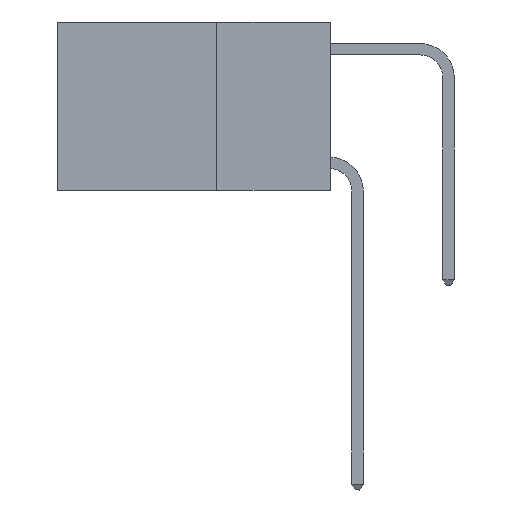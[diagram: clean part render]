
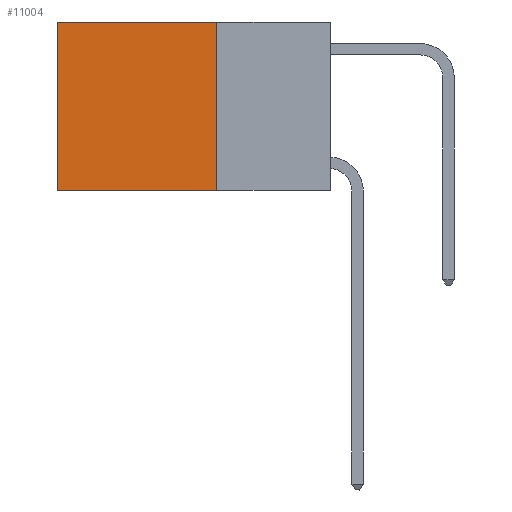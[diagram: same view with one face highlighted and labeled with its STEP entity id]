
A CAD part, left-side view. The second image highlights one B-rep face of the part: STEP entity #11004.
In plain terms, the highlighted planar face has unit normal (-1, 0, 0).
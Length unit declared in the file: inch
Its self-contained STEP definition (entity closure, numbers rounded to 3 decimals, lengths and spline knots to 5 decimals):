
#672 = DIRECTION ( 'NONE',  ( 0., 1., 0. ) ) ;
#1642 = DIRECTION ( 'NONE',  ( 0., 0., -1. ) ) ;
#2184 = VECTOR ( 'NONE', #5513, 39.37008 ) ;
#2373 = VECTOR ( 'NONE', #6377, 39.37008 ) ;
#2570 = PLANE ( 'NONE',  #9098 ) ;
#2979 = VECTOR ( 'NONE', #1642, 39.37008 ) ;
#3345 = VERTEX_POINT ( 'NONE', #8348 ) ;
#3368 = CARTESIAN_POINT ( 'NONE',  ( 0.2625, 0.6, 0. ) ) ;
#3520 = VERTEX_POINT ( 'NONE', #6360 ) ;
#3908 = ORIENTED_EDGE ( 'NONE', *, *, #7059, .F. ) ;
#4162 = EDGE_LOOP ( 'NONE', ( #11677, #3908, #10853, #10367 ) ) ;
#4554 = CARTESIAN_POINT ( 'NONE',  ( 0.2625, 0.6, 0. ) ) ;
#5513 = DIRECTION ( 'NONE',  ( 0., 0., -1. ) ) ;
#5763 = CARTESIAN_POINT ( 'NONE',  ( 0.2625, 0.25, 0. ) ) ;
#5801 = LINE ( 'NONE', #6273, #2979 ) ;
#6016 = EDGE_CURVE ( 'NONE', #13277, #3520, #5801, .T. ) ;
#6273 = CARTESIAN_POINT ( 'NONE',  ( 0.2625, 0.25, 0. ) ) ;
#6360 = CARTESIAN_POINT ( 'NONE',  ( 0.2625, 0.25, -0.37 ) ) ;
#6377 = DIRECTION ( 'NONE',  ( 0., 1., 0. ) ) ;
#6893 = CARTESIAN_POINT ( 'NONE',  ( 0.2625, 0.25, -0.37 ) ) ;
#7059 = EDGE_CURVE ( 'NONE', #3520, #3345, #12704, .T. ) ;
#7396 = CARTESIAN_POINT ( 'NONE',  ( 0.2625, 0.25, 0. ) ) ;
#8348 = CARTESIAN_POINT ( 'NONE',  ( 0.2625, 0.6, -0.37 ) ) ;
#9098 = AXIS2_PLACEMENT_3D ( 'NONE', #11975, #12250, #11227 ) ;
#9104 = VECTOR ( 'NONE', #672, 39.37008 ) ;
#10367 = ORIENTED_EDGE ( 'NONE', *, *, #12361, .T. ) ;
#10629 = LINE ( 'NONE', #3368, #2184 ) ;
#10848 = EDGE_CURVE ( 'NONE', #12569, #3345, #10629, .T. ) ;
#10853 = ORIENTED_EDGE ( 'NONE', *, *, #6016, .F. ) ;
#11004 = ADVANCED_FACE ( 'NONE', ( #11799 ), #2570, .F. ) ;
#11144 = LINE ( 'NONE', #7396, #2373 ) ;
#11227 = DIRECTION ( 'NONE',  ( 0., 0., -1. ) ) ;
#11677 = ORIENTED_EDGE ( 'NONE', *, *, #10848, .T. ) ;
#11799 = FACE_OUTER_BOUND ( 'NONE', #4162, .T. ) ;
#11975 = CARTESIAN_POINT ( 'NONE',  ( 0.2625, 0.25, 0. ) ) ;
#12250 = DIRECTION ( 'NONE',  ( 1., 0., 0. ) ) ;
#12361 = EDGE_CURVE ( 'NONE', #13277, #12569, #11144, .T. ) ;
#12569 = VERTEX_POINT ( 'NONE', #4554 ) ;
#12704 = LINE ( 'NONE', #6893, #9104 ) ;
#13277 = VERTEX_POINT ( 'NONE', #5763 ) ;
